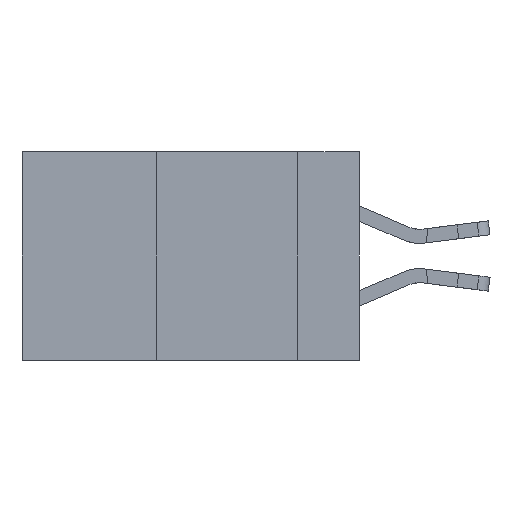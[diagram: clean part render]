
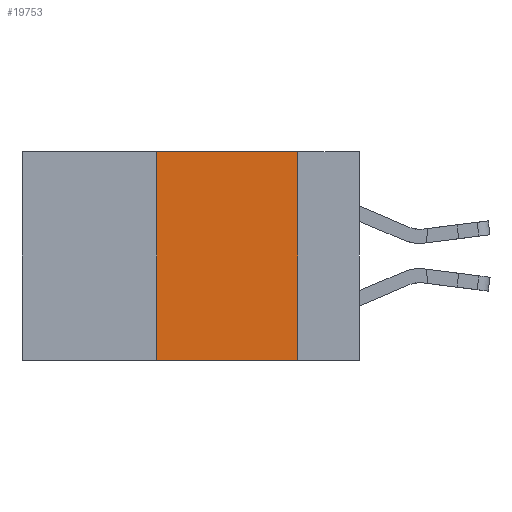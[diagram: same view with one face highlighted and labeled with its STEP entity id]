
A CAD part, left-side view. The second image highlights one B-rep face of the part: STEP entity #19753.
In plain terms, the highlighted planar face has unit normal (-1, 0, 0).
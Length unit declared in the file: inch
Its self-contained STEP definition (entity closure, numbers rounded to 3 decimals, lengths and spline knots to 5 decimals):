
#126 = LINE ( 'NONE', #6044, #14527 ) ;
#2535 = DIRECTION ( 'NONE',  ( 0., 0., 1. ) ) ;
#3991 = CARTESIAN_POINT ( 'NONE',  ( 0., 0.6, 0. ) ) ;
#4047 = VERTEX_POINT ( 'NONE', #7658 ) ;
#4387 = CARTESIAN_POINT ( 'NONE',  ( 0., 0.11, 0. ) ) ;
#4717 = CARTESIAN_POINT ( 'NONE',  ( 0., 0.6, -0.37 ) ) ;
#6044 = CARTESIAN_POINT ( 'NONE',  ( 0., 0.36, 0. ) ) ;
#6212 = ORIENTED_EDGE ( 'NONE', *, *, #24202, .F. ) ;
#7658 = CARTESIAN_POINT ( 'NONE',  ( 0., 0.36, 0. ) ) ;
#7864 = EDGE_CURVE ( 'NONE', #21697, #23398, #14961, .T. ) ;
#9194 = ORIENTED_EDGE ( 'NONE', *, *, #11426, .F. ) ;
#9218 = ORIENTED_EDGE ( 'NONE', *, *, #16746, .F. ) ;
#10447 = DIRECTION ( 'NONE',  ( 0., -1., 0. ) ) ;
#11426 = EDGE_CURVE ( 'NONE', #21652, #23398, #17164, .T. ) ;
#11617 = DIRECTION ( 'NONE',  ( 0., 0., -1. ) ) ;
#11875 = PLANE ( 'NONE',  #21957 ) ;
#12458 = CARTESIAN_POINT ( 'NONE',  ( 0., 0.6, 0. ) ) ;
#13549 = LINE ( 'NONE', #3991, #24159 ) ;
#13636 = CARTESIAN_POINT ( 'NONE',  ( 0., 0.11, -0.37 ) ) ;
#13998 = CARTESIAN_POINT ( 'NONE',  ( 0., 0.11, 0. ) ) ;
#14333 = DIRECTION ( 'NONE',  ( 0., 0., -1. ) ) ;
#14527 = VECTOR ( 'NONE', #2535, 39.37008 ) ;
#14961 = LINE ( 'NONE', #4717, #21781 ) ;
#15381 = DIRECTION ( 'NONE',  ( 0., -1., 0. ) ) ;
#16746 = EDGE_CURVE ( 'NONE', #4047, #21652, #13549, .T. ) ;
#17164 = LINE ( 'NONE', #4387, #18350 ) ;
#18350 = VECTOR ( 'NONE', #11617, 39.37008 ) ;
#19659 = FACE_OUTER_BOUND ( 'NONE', #21031, .T. ) ;
#19753 = ADVANCED_FACE ( 'NONE', ( #19659 ), #11875, .F. ) ;
#20190 = CARTESIAN_POINT ( 'NONE',  ( 0., 0.36, -0.37 ) ) ;
#20220 = ORIENTED_EDGE ( 'NONE', *, *, #7864, .T. ) ;
#21031 = EDGE_LOOP ( 'NONE', ( #9194, #9218, #6212, #20220 ) ) ;
#21652 = VERTEX_POINT ( 'NONE', #13998 ) ;
#21697 = VERTEX_POINT ( 'NONE', #20190 ) ;
#21781 = VECTOR ( 'NONE', #10447, 39.37008 ) ;
#21856 = DIRECTION ( 'NONE',  ( 1., 0., 0. ) ) ;
#21957 = AXIS2_PLACEMENT_3D ( 'NONE', #12458, #21856, #14333 ) ;
#23398 = VERTEX_POINT ( 'NONE', #13636 ) ;
#24159 = VECTOR ( 'NONE', #15381, 39.37008 ) ;
#24202 = EDGE_CURVE ( 'NONE', #21697, #4047, #126, .T. ) ;
